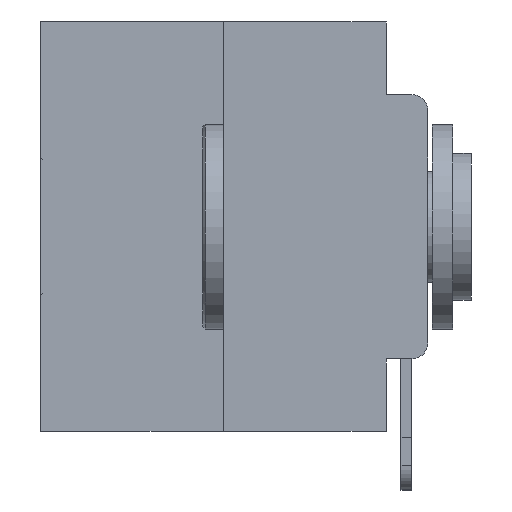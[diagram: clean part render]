
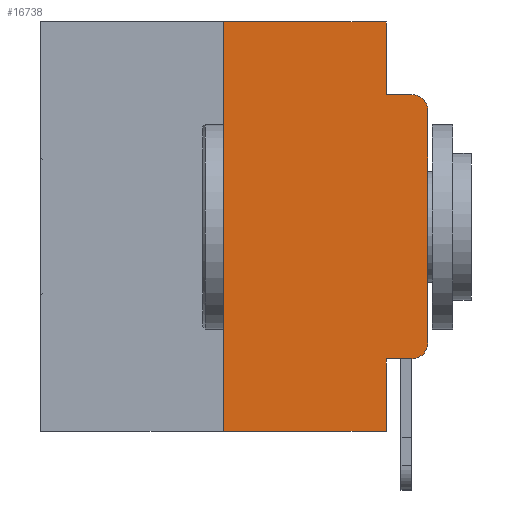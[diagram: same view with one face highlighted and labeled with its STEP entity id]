
A CAD part, left-side view. The second image highlights one B-rep face of the part: STEP entity #16738.
In plain terms, the highlighted planar face has unit normal (-1, 0, 0).
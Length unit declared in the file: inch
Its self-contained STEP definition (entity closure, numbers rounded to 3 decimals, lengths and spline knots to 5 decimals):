
#10 = ORIENTED_EDGE ( 'NONE', *, *, #6421, .T. ) ;
#56 = LINE ( 'NONE', #20606, #23946 ) ;
#243 = VERTEX_POINT ( 'NONE', #21691 ) ;
#408 = LINE ( 'NONE', #21916, #1909 ) ;
#1306 = CARTESIAN_POINT ( 'NONE',  ( 0., 0.02, -0.3915 ) ) ;
#1343 = ORIENTED_EDGE ( 'NONE', *, *, #2726, .T. ) ;
#1383 = VERTEX_POINT ( 'NONE', #17663 ) ;
#1437 = DIRECTION ( 'NONE',  ( 0., 0., -1. ) ) ;
#1909 = VECTOR ( 'NONE', #24178, 39.37008 ) ;
#2026 = DIRECTION ( 'NONE',  ( 0., -1., 0. ) ) ;
#2536 = ORIENTED_EDGE ( 'NONE', *, *, #24700, .F. ) ;
#2726 = EDGE_CURVE ( 'NONE', #24543, #5028, #17881, .T. ) ;
#3179 = ORIENTED_EDGE ( 'NONE', *, *, #29756, .F. ) ;
#3473 = VERTEX_POINT ( 'NONE', #23446 ) ;
#3689 = DIRECTION ( 'NONE',  ( 0., 0., -1. ) ) ;
#3718 = DIRECTION ( 'NONE',  ( 0., 0., -1. ) ) ;
#4142 = DIRECTION ( 'NONE',  ( 0., -1., 0. ) ) ;
#4278 = AXIS2_PLACEMENT_3D ( 'NONE', #1306, #17546, #3718 ) ;
#5028 = VERTEX_POINT ( 'NONE', #5338 ) ;
#5338 = CARTESIAN_POINT ( 'NONE',  ( 0., 0.02, -0.4115 ) ) ;
#5525 = EDGE_CURVE ( 'NONE', #1383, #243, #28024, .T. ) ;
#5917 = EDGE_CURVE ( 'NONE', #17068, #3473, #12750, .T. ) ;
#5960 = PLANE ( 'NONE',  #8830 ) ;
#6421 = EDGE_CURVE ( 'NONE', #5028, #29097, #24115, .T. ) ;
#6565 = DIRECTION ( 'NONE',  ( 0., 0., -1. ) ) ;
#7839 = CARTESIAN_POINT ( 'NONE',  ( 0., 0.25, -0.5 ) ) ;
#8084 = ORIENTED_EDGE ( 'NONE', *, *, #14043, .F. ) ;
#8479 = VERTEX_POINT ( 'NONE', #12646 ) ;
#8728 = CARTESIAN_POINT ( 'NONE',  ( 0., 0., -0.1085 ) ) ;
#8830 = AXIS2_PLACEMENT_3D ( 'NONE', #26588, #17519, #3689 ) ;
#9890 = VECTOR ( 'NONE', #20818, 39.37008 ) ;
#10648 = CARTESIAN_POINT ( 'NONE',  ( 0., 0.051, -0.4115 ) ) ;
#11290 = VECTOR ( 'NONE', #4142, 39.37008 ) ;
#12093 = ORIENTED_EDGE ( 'NONE', *, *, #5917, .T. ) ;
#12563 = LINE ( 'NONE', #14826, #29208 ) ;
#12646 = CARTESIAN_POINT ( 'NONE',  ( 0., 0.051, -0.0885 ) ) ;
#12750 = CIRCLE ( 'NONE', #13223, 0.02 ) ;
#13096 = ORIENTED_EDGE ( 'NONE', *, *, #18985, .F. ) ;
#13223 = AXIS2_PLACEMENT_3D ( 'NONE', #28960, #15385, #1437 ) ;
#13404 = ORIENTED_EDGE ( 'NONE', *, *, #5525, .F. ) ;
#14043 = EDGE_CURVE ( 'NONE', #8479, #3473, #17342, .T. ) ;
#14458 = ORIENTED_EDGE ( 'NONE', *, *, #23409, .T. ) ;
#14826 = CARTESIAN_POINT ( 'NONE',  ( 0., 0.473, -0.5 ) ) ;
#15385 = DIRECTION ( 'NONE',  ( -1., 0., 0. ) ) ;
#16200 = CARTESIAN_POINT ( 'NONE',  ( 0., 0.473, 0. ) ) ;
#16717 = CARTESIAN_POINT ( 'NONE',  ( 0., 0.051, -0.5 ) ) ;
#16738 = ADVANCED_FACE ( 'NONE', ( #21205 ), #5960, .F. ) ;
#17068 = VERTEX_POINT ( 'NONE', #8728 ) ;
#17342 = LINE ( 'NONE', #17975, #11290 ) ;
#17519 = DIRECTION ( 'NONE',  ( 1., 0., 0. ) ) ;
#17546 = DIRECTION ( 'NONE',  ( -1., 0., 0. ) ) ;
#17663 = CARTESIAN_POINT ( 'NONE',  ( 0., 0.25, 0. ) ) ;
#17881 = LINE ( 'NONE', #24542, #29196 ) ;
#17975 = CARTESIAN_POINT ( 'NONE',  ( 0., 0.051, -0.0885 ) ) ;
#18135 = VERTEX_POINT ( 'NONE', #7839 ) ;
#18205 = VECTOR ( 'NONE', #6565, 39.37008 ) ;
#18548 = VERTEX_POINT ( 'NONE', #16717 ) ;
#18813 = DIRECTION ( 'NONE',  ( 0., 0., 1. ) ) ;
#18985 = EDGE_CURVE ( 'NONE', #24543, #18548, #56, .T. ) ;
#19848 = ORIENTED_EDGE ( 'NONE', *, *, #28852, .T. ) ;
#20435 = LINE ( 'NONE', #23407, #25751 ) ;
#20606 = CARTESIAN_POINT ( 'NONE',  ( 0., 0.051, 0. ) ) ;
#20818 = DIRECTION ( 'NONE',  ( 0., -1., 0. ) ) ;
#21205 = FACE_OUTER_BOUND ( 'NONE', #29795, .T. ) ;
#21691 = CARTESIAN_POINT ( 'NONE',  ( 0., 0.051, 0. ) ) ;
#21735 = DIRECTION ( 'NONE',  ( 0., -1., 0. ) ) ;
#21916 = CARTESIAN_POINT ( 'NONE',  ( 0., 0.25, 0. ) ) ;
#22011 = CARTESIAN_POINT ( 'NONE',  ( 0., 0., -0.3915 ) ) ;
#23407 = CARTESIAN_POINT ( 'NONE',  ( 0., 0., 0. ) ) ;
#23409 = EDGE_CURVE ( 'NONE', #18135, #18548, #12563, .T. ) ;
#23446 = CARTESIAN_POINT ( 'NONE',  ( 0., 0.02, -0.0885 ) ) ;
#23946 = VECTOR ( 'NONE', #25158, 39.37008 ) ;
#24115 = CIRCLE ( 'NONE', #4278, 0.02 ) ;
#24178 = DIRECTION ( 'NONE',  ( 0., 0., 1. ) ) ;
#24265 = LINE ( 'NONE', #27060, #18205 ) ;
#24542 = CARTESIAN_POINT ( 'NONE',  ( 0., 0.051, -0.4115 ) ) ;
#24543 = VERTEX_POINT ( 'NONE', #10648 ) ;
#24700 = EDGE_CURVE ( 'NONE', #243, #8479, #24265, .T. ) ;
#25158 = DIRECTION ( 'NONE',  ( 0., 0., -1. ) ) ;
#25751 = VECTOR ( 'NONE', #18813, 39.37008 ) ;
#26588 = CARTESIAN_POINT ( 'NONE',  ( 0., 0.473, 0. ) ) ;
#27060 = CARTESIAN_POINT ( 'NONE',  ( 0., 0.051, 0. ) ) ;
#28024 = LINE ( 'NONE', #16200, #9890 ) ;
#28852 = EDGE_CURVE ( 'NONE', #29097, #17068, #20435, .T. ) ;
#28960 = CARTESIAN_POINT ( 'NONE',  ( 0., 0.02, -0.1085 ) ) ;
#29097 = VERTEX_POINT ( 'NONE', #22011 ) ;
#29196 = VECTOR ( 'NONE', #2026, 39.37008 ) ;
#29208 = VECTOR ( 'NONE', #21735, 39.37008 ) ;
#29756 = EDGE_CURVE ( 'NONE', #18135, #1383, #408, .T. ) ;
#29795 = EDGE_LOOP ( 'NONE', ( #19848, #12093, #8084, #2536, #13404, #3179, #14458, #13096, #1343, #10 ) ) ;
